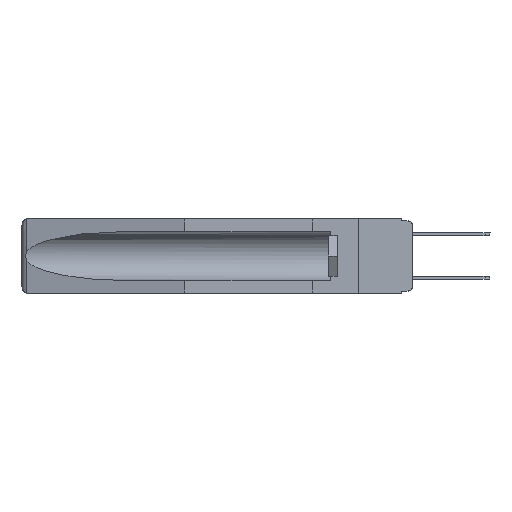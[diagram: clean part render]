
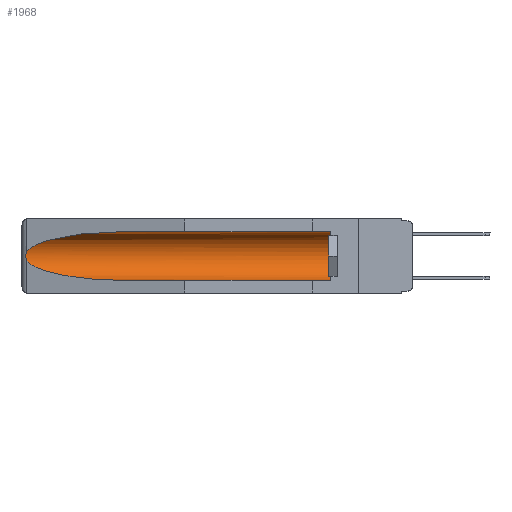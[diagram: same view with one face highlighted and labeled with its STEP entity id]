
A CAD part, left-side view. The second image highlights one B-rep face of the part: STEP entity #1968.
In plain terms, the highlighted cylindrical face has radius 2.857 mm (diameter 5.715 mm), a partial arc.
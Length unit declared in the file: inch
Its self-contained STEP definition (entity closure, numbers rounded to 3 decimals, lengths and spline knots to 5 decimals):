
#39 = FACE_OUTER_BOUND ( 'NONE', #13263, .T. ) ;
#53 = ORIENTED_EDGE ( 'NONE', *, *, #16370, .T. ) ;
#114 = CARTESIAN_POINT ( 'NONE',  ( 0.26537, 1.52718, -0.14972 ) ) ;
#131 = CARTESIAN_POINT ( 'NONE',  ( 0.25451, 1.48313, -0.09465 ) ) ;
#641 = CIRCLE ( 'NONE', #9448, 0.1125 ) ;
#844 = CARTESIAN_POINT ( 'NONE',  ( 0.2673, 1.5327, -0.16383 ) ) ;
#928 = CARTESIAN_POINT ( 'NONE',  ( 0.2675, 1.53308, -0.17534 ) ) ;
#993 = CARTESIAN_POINT ( 'NONE',  ( 0.21114, 1.30732, -0.284 ) ) ;
#1192 = DIRECTION ( 'NONE',  ( 0., 0., 1. ) ) ;
#1746 = VERTEX_POINT ( 'NONE', #7346 ) ;
#1968 = ADVANCED_FACE ( 'NONE', ( #39 ), #12121, .F. ) ;
#2066 = CARTESIAN_POINT ( 'NONE',  ( 0.155, -0.30754, -0.284 ) ) ;
#2231 = B_SPLINE_CURVE_WITH_KNOTS ( 'NONE', 3,
 ( #14358, #7598, #13012, #844, #6279, #928, #11691, #6365, #17204, #5033 ),
 .UNSPECIFIED., .F., .F.,
 ( 4, 2, 2, 2, 4 ),
 ( 0., 0.00029, 0.00058, 0.00087, 0.00117 ),
 .UNSPECIFIED. ) ;
#2336 = ORIENTED_EDGE ( 'NONE', *, *, #15059, .T. ) ;
#2405 = EDGE_CURVE ( 'NONE', #10381, #15203, #641, .T. ) ;
#2610 = DIRECTION ( 'NONE',  ( 0., 1., 0. ) ) ;
#3344 = EDGE_CURVE ( 'NONE', #1746, #12557, #12649, .T. ) ;
#3745 = ORIENTED_EDGE ( 'NONE', *, *, #2405, .T. ) ;
#5033 = CARTESIAN_POINT ( 'NONE',  ( 0.26537, 1.52718, -0.19328 ) ) ;
#5251 = DIRECTION ( 'NONE',  ( 0., -1., 0. ) ) ;
#5375 = CARTESIAN_POINT ( 'NONE',  ( 0.26537, 1.52718, -0.14972 ) ) ;
#5858 = CARTESIAN_POINT ( 'NONE',  ( 0.155, 1.07973, -0.284 ) ) ;
#6088 = EDGE_CURVE ( 'NONE', #10381, #16071, #12907, .T. ) ;
#6188 = ORIENTED_EDGE ( 'NONE', *, *, #3344, .T. ) ;
#6279 = CARTESIAN_POINT ( 'NONE',  ( 0.2675, 1.53308, -0.16763 ) ) ;
#6365 = CARTESIAN_POINT ( 'NONE',  ( 0.26655, 1.53094, -0.18657 ) ) ;
#7346 = CARTESIAN_POINT ( 'NONE',  ( 0.155, 1.07973, -0.059 ) ) ;
#7598 = CARTESIAN_POINT ( 'NONE',  ( 0.26597, 1.52961, -0.15275 ) ) ;
#7939 = CARTESIAN_POINT ( 'NONE',  ( 0.21114, 1.30732, -0.059 ) ) ;
#8030 = DIRECTION ( 'NONE',  ( 0., 1., 0. ) ) ;
#8140 = CARTESIAN_POINT ( 'NONE',  ( 0.155, 1.07973, -0.284 ) ) ;
#8573 = ORIENTED_EDGE ( 'NONE', *, *, #6088, .F. ) ;
#9347 = EDGE_CURVE ( 'NONE', #13453, #16071, #14474, .T. ) ;
#9448 = AXIS2_PLACEMENT_3D ( 'NONE', #12004, #5251, #14754 ) ;
#9996 = AXIS2_PLACEMENT_3D ( 'NONE', #13266, #2610, #1192 ) ;
#10037 = CARTESIAN_POINT ( 'NONE',  ( 0.155, 0.126, -0.284 ) ) ;
#10381 = VERTEX_POINT ( 'NONE', #10037 ) ;
#10514 = LINE ( 'NONE', #16316, #16988 ) ;
#10974 = CARTESIAN_POINT ( 'NONE',  ( 0.26537, 1.52718, -0.19328 ) ) ;
#11691 = CARTESIAN_POINT ( 'NONE',  ( 0.2673, 1.53269, -0.17917 ) ) ;
#11959 = CARTESIAN_POINT ( 'NONE',  ( 0.155, 1.07973, -0.059 ) ) ;
#12004 = CARTESIAN_POINT ( 'NONE',  ( 0.155, 0.126, -0.1715 ) ) ;
#12061 = VECTOR ( 'NONE', #16681, 39.37008 ) ;
#12121 = CYLINDRICAL_SURFACE ( 'NONE', #9996, 0.1125 ) ;
#12557 = VERTEX_POINT ( 'NONE', #114 ) ;
#12649 =( BOUNDED_CURVE ( )  B_SPLINE_CURVE ( 3, ( #11959, #7939, #131, #5375 ),
 .UNSPECIFIED., .F., .T. ) 
 B_SPLINE_CURVE_WITH_KNOTS ( ( 4, 4 ),
 ( 4.71239, 6.08839 ),
 .UNSPECIFIED. ) 
 CURVE ( )  GEOMETRIC_REPRESENTATION_ITEM ( )  RATIONAL_B_SPLINE_CURVE ( ( 1., 0.848, 0.848, 1. ) ) 
 REPRESENTATION_ITEM ( '' )  );
#12907 = LINE ( 'NONE', #2066, #12061 ) ;
#13012 = CARTESIAN_POINT ( 'NONE',  ( 0.26654, 1.53092, -0.15636 ) ) ;
#13263 = EDGE_LOOP ( 'NONE', ( #6188, #53, #14080, #8573, #3745, #2336 ) ) ;
#13266 = CARTESIAN_POINT ( 'NONE',  ( 0.155, -0.30754, -0.1715 ) ) ;
#13453 = VERTEX_POINT ( 'NONE', #17003 ) ;
#13613 = CARTESIAN_POINT ( 'NONE',  ( 0.155, 0.126, -0.059 ) ) ;
#14080 = ORIENTED_EDGE ( 'NONE', *, *, #9347, .T. ) ;
#14358 = CARTESIAN_POINT ( 'NONE',  ( 0.26537, 1.52718, -0.14972 ) ) ;
#14474 =( BOUNDED_CURVE ( )  B_SPLINE_CURVE ( 3, ( #10974, #17189, #993, #5858 ),
 .UNSPECIFIED., .F., .F. ) 
 B_SPLINE_CURVE_WITH_KNOTS ( ( 4, 4 ),
 ( 0.1948, 1.5708 ),
 .UNSPECIFIED. ) 
 CURVE ( )  GEOMETRIC_REPRESENTATION_ITEM ( )  RATIONAL_B_SPLINE_CURVE ( ( 1., 0.848, 0.848, 1. ) ) 
 REPRESENTATION_ITEM ( '' )  );
#14754 = DIRECTION ( 'NONE',  ( 0., 0., 1. ) ) ;
#15059 = EDGE_CURVE ( 'NONE', #15203, #1746, #10514, .T. ) ;
#15203 = VERTEX_POINT ( 'NONE', #13613 ) ;
#16071 = VERTEX_POINT ( 'NONE', #8140 ) ;
#16316 = CARTESIAN_POINT ( 'NONE',  ( 0.155, -0.30754, -0.059 ) ) ;
#16370 = EDGE_CURVE ( 'NONE', #12557, #13453, #2231, .T. ) ;
#16681 = DIRECTION ( 'NONE',  ( 0., 1., 0. ) ) ;
#16988 = VECTOR ( 'NONE', #8030, 39.37008 ) ;
#17003 = CARTESIAN_POINT ( 'NONE',  ( 0.26537, 1.52718, -0.19328 ) ) ;
#17189 = CARTESIAN_POINT ( 'NONE',  ( 0.25451, 1.48313, -0.24835 ) ) ;
#17204 = CARTESIAN_POINT ( 'NONE',  ( 0.26597, 1.5296, -0.19026 ) ) ;
